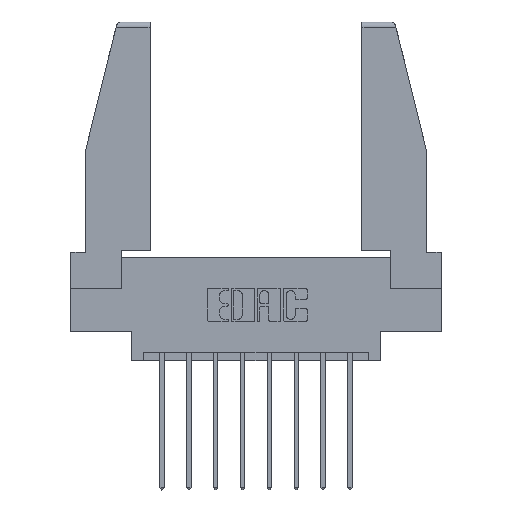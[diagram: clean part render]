
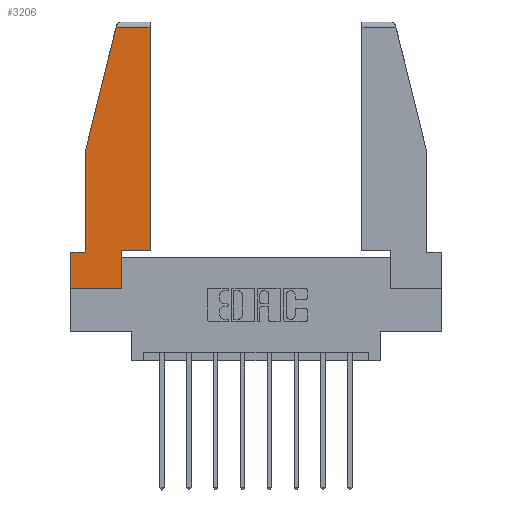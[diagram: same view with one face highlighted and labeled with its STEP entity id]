
A CAD part, top view. The second image highlights one B-rep face of the part: STEP entity #3206.
In plain terms, the highlighted planar face has unit normal (0, 0, 1).
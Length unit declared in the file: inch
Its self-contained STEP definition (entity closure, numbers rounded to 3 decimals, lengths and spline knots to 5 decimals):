
#48 = CARTESIAN_POINT ( 'NONE',  ( 0.297, 0., 0. ) ) ;
#944 = LINE ( 'NONE', #7082, #10694 ) ;
#1123 = EDGE_CURVE ( 'NONE', #2689, #2319, #11652, .T. ) ;
#1259 = CARTESIAN_POINT ( 'NONE',  ( 0., 0., 0. ) ) ;
#1397 = DIRECTION ( 'NONE',  ( 1., 0., 0. ) ) ;
#1497 = ORIENTED_EDGE ( 'NONE', *, *, #12107, .T. ) ;
#1734 = CARTESIAN_POINT ( 'NONE',  ( 0., 1.52, 0. ) ) ;
#2101 = VECTOR ( 'NONE', #1397, 39.37008 ) ;
#2257 = DIRECTION ( 'NONE',  ( 1., 0., 0. ) ) ;
#2319 = VERTEX_POINT ( 'NONE', #3025 ) ;
#2423 = VERTEX_POINT ( 'NONE', #4395 ) ;
#2433 = FACE_OUTER_BOUND ( 'NONE', #4540, .T. ) ;
#2545 = ORIENTED_EDGE ( 'NONE', *, *, #1123, .T. ) ;
#2689 = VERTEX_POINT ( 'NONE', #10833 ) ;
#3025 = CARTESIAN_POINT ( 'NONE',  ( 0.086, 0.21, 0. ) ) ;
#3073 = EDGE_CURVE ( 'NONE', #6489, #2423, #8526, .T. ) ;
#3206 = ADVANCED_FACE ( 'NONE', ( #2433 ), #9406, .T. ) ;
#3434 = AXIS2_PLACEMENT_3D ( 'NONE', #11445, #10515, #2257 ) ;
#4076 = EDGE_CURVE ( 'NONE', #2423, #2689, #7523, .T. ) ;
#4395 = CARTESIAN_POINT ( 'NONE',  ( 0.2636, 1.52, 0. ) ) ;
#4405 = VECTOR ( 'NONE', #8737, 39.37008 ) ;
#4462 = LINE ( 'NONE', #11403, #6873 ) ;
#4540 = EDGE_LOOP ( 'NONE', ( #11845, #11313, #11167, #2545, #8726, #1497, #7340, #8386, #6509 ) ) ;
#4586 = VECTOR ( 'NONE', #9055, 39.37008 ) ;
#4716 = DIRECTION ( 'NONE',  ( -0.239, -0.971, 0. ) ) ;
#4897 = VERTEX_POINT ( 'NONE', #48 ) ;
#5121 = CARTESIAN_POINT ( 'NONE',  ( 0.461, 0.223, 0. ) ) ;
#5190 = CARTESIAN_POINT ( 'NONE',  ( 0.297, 0.223, 0. ) ) ;
#5294 = LINE ( 'NONE', #5121, #6261 ) ;
#5582 = VECTOR ( 'NONE', #4716, 39.37008 ) ;
#5734 = DIRECTION ( 'NONE',  ( -1., 0., 0. ) ) ;
#6083 = DIRECTION ( 'NONE',  ( 1., 0., 0. ) ) ;
#6165 = VERTEX_POINT ( 'NONE', #12894 ) ;
#6261 = VECTOR ( 'NONE', #8266, 39.37008 ) ;
#6299 = DIRECTION ( 'NONE',  ( 0., 1., 0. ) ) ;
#6489 = VERTEX_POINT ( 'NONE', #10583 ) ;
#6509 = ORIENTED_EDGE ( 'NONE', *, *, #11562, .T. ) ;
#6678 = VECTOR ( 'NONE', #11904, 39.37008 ) ;
#6857 = LINE ( 'NONE', #13120, #6678 ) ;
#6873 = VECTOR ( 'NONE', #6299, 39.37008 ) ;
#7082 = CARTESIAN_POINT ( 'NONE',  ( 0.297, 0.223, 0. ) ) ;
#7305 = CARTESIAN_POINT ( 'NONE',  ( 0., 0.21, 0. ) ) ;
#7340 = ORIENTED_EDGE ( 'NONE', *, *, #10277, .T. ) ;
#7523 = LINE ( 'NONE', #11837, #5582 ) ;
#7601 = CARTESIAN_POINT ( 'NONE',  ( 0., 0.21, 0. ) ) ;
#7682 = CARTESIAN_POINT ( 'NONE',  ( 0.461, 0.223, 0. ) ) ;
#7877 = VECTOR ( 'NONE', #5734, 39.37008 ) ;
#8266 = DIRECTION ( 'NONE',  ( 0., 1., 0. ) ) ;
#8386 = ORIENTED_EDGE ( 'NONE', *, *, #11111, .T. ) ;
#8526 = LINE ( 'NONE', #1734, #7877 ) ;
#8726 = ORIENTED_EDGE ( 'NONE', *, *, #11628, .T. ) ;
#8737 = DIRECTION ( 'NONE',  ( 0., -1., 0. ) ) ;
#8789 = VERTEX_POINT ( 'NONE', #7682 ) ;
#9055 = DIRECTION ( 'NONE',  ( 0., -1., 0. ) ) ;
#9225 = LINE ( 'NONE', #7601, #4405 ) ;
#9233 = VERTEX_POINT ( 'NONE', #5190 ) ;
#9406 = PLANE ( 'NONE',  #3434 ) ;
#10029 = EDGE_CURVE ( 'NONE', #8789, #6489, #5294, .T. ) ;
#10265 = LINE ( 'NONE', #1259, #2101 ) ;
#10277 = EDGE_CURVE ( 'NONE', #6165, #4897, #10265, .T. ) ;
#10515 = DIRECTION ( 'NONE',  ( 0., 0., 1. ) ) ;
#10583 = CARTESIAN_POINT ( 'NONE',  ( 0.461, 1.52, 0. ) ) ;
#10694 = VECTOR ( 'NONE', #6083, 39.37008 ) ;
#10833 = CARTESIAN_POINT ( 'NONE',  ( 0.086, 0.8, 0. ) ) ;
#11111 = EDGE_CURVE ( 'NONE', #4897, #9233, #4462, .T. ) ;
#11167 = ORIENTED_EDGE ( 'NONE', *, *, #4076, .T. ) ;
#11313 = ORIENTED_EDGE ( 'NONE', *, *, #3073, .T. ) ;
#11403 = CARTESIAN_POINT ( 'NONE',  ( 0.297, 0., 0. ) ) ;
#11445 = CARTESIAN_POINT ( 'NONE',  ( 0., 0., 0. ) ) ;
#11562 = EDGE_CURVE ( 'NONE', #9233, #8789, #944, .T. ) ;
#11603 = VERTEX_POINT ( 'NONE', #7305 ) ;
#11628 = EDGE_CURVE ( 'NONE', #2319, #11603, #6857, .T. ) ;
#11652 = LINE ( 'NONE', #13122, #4586 ) ;
#11837 = CARTESIAN_POINT ( 'NONE',  ( 0.271, 1.55, 0. ) ) ;
#11845 = ORIENTED_EDGE ( 'NONE', *, *, #10029, .T. ) ;
#11904 = DIRECTION ( 'NONE',  ( -1., 0., 0. ) ) ;
#12107 = EDGE_CURVE ( 'NONE', #11603, #6165, #9225, .T. ) ;
#12894 = CARTESIAN_POINT ( 'NONE',  ( 0., 0., 0. ) ) ;
#13120 = CARTESIAN_POINT ( 'NONE',  ( 0., 0.21, 0. ) ) ;
#13122 = CARTESIAN_POINT ( 'NONE',  ( 0.086, 0.8, 0. ) ) ;
